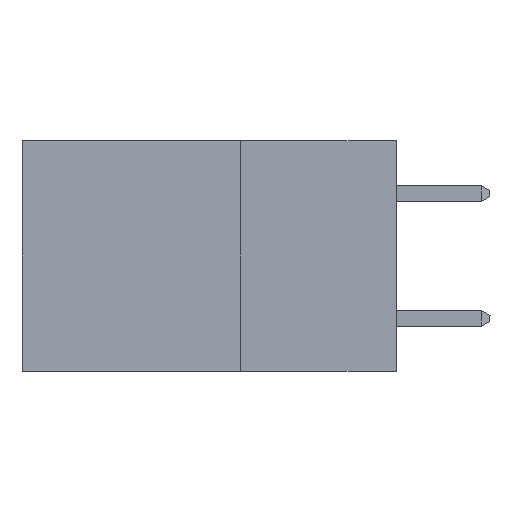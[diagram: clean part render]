
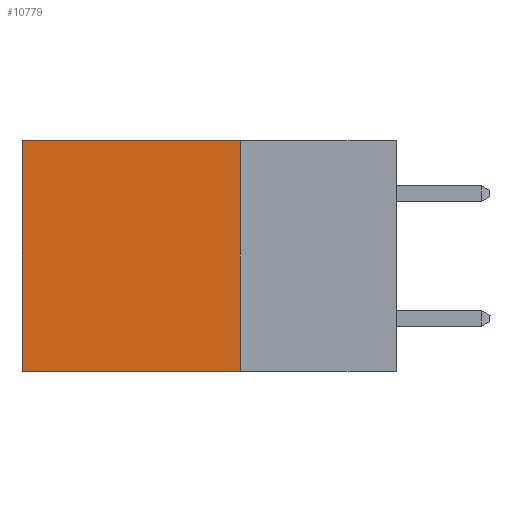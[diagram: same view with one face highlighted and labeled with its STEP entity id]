
A CAD part, left-side view. The second image highlights one B-rep face of the part: STEP entity #10779.
In plain terms, the highlighted planar face has unit normal (-1, 0, 0).
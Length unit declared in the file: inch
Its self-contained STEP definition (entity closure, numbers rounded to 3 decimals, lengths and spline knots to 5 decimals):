
#13 = PLANE ( 'NONE',  #3113 ) ;
#426 = CARTESIAN_POINT ( 'NONE',  ( 0.298, 0.6, 0. ) ) ;
#3113 = AXIS2_PLACEMENT_3D ( 'NONE', #16318, #10113, #12138 ) ;
#3839 = VECTOR ( 'NONE', #6429, 39.37008 ) ;
#4372 = LINE ( 'NONE', #426, #19845 ) ;
#5402 = ORIENTED_EDGE ( 'NONE', *, *, #8547, .F. ) ;
#5595 = VERTEX_POINT ( 'NONE', #21946 ) ;
#5607 = EDGE_CURVE ( 'NONE', #5595, #17374, #20962, .T. ) ;
#6304 = EDGE_LOOP ( 'NONE', ( #10473, #5402, #8585, #14293 ) ) ;
#6429 = DIRECTION ( 'NONE',  ( 0., 1., 0. ) ) ;
#6780 = CARTESIAN_POINT ( 'NONE',  ( 0.298, 0.25, -0.37 ) ) ;
#7233 = FACE_OUTER_BOUND ( 'NONE', #6304, .T. ) ;
#7769 = CARTESIAN_POINT ( 'NONE',  ( 0.298, 0.6, 0. ) ) ;
#8212 = VECTOR ( 'NONE', #14818, 39.37008 ) ;
#8547 = EDGE_CURVE ( 'NONE', #22191, #12712, #25007, .T. ) ;
#8585 = ORIENTED_EDGE ( 'NONE', *, *, #25036, .F. ) ;
#10113 = DIRECTION ( 'NONE',  ( 1., 0., 0. ) ) ;
#10473 = ORIENTED_EDGE ( 'NONE', *, *, #18864, .T. ) ;
#10779 = ADVANCED_FACE ( 'NONE', ( #7233 ), #13, .F. ) ;
#12138 = DIRECTION ( 'NONE',  ( 0., 0., -1. ) ) ;
#12712 = VERTEX_POINT ( 'NONE', #21844 ) ;
#12806 = DIRECTION ( 'NONE',  ( 0., 0., -1. ) ) ;
#12925 = CARTESIAN_POINT ( 'NONE',  ( 0.298, 0.25, 0. ) ) ;
#14293 = ORIENTED_EDGE ( 'NONE', *, *, #5607, .T. ) ;
#14818 = DIRECTION ( 'NONE',  ( 0., 0., -1. ) ) ;
#16318 = CARTESIAN_POINT ( 'NONE',  ( 0.298, 0.25, 0. ) ) ;
#17374 = VERTEX_POINT ( 'NONE', #7769 ) ;
#18864 = EDGE_CURVE ( 'NONE', #17374, #12712, #4372, .T. ) ;
#19832 = DIRECTION ( 'NONE',  ( 0., 1., 0. ) ) ;
#19845 = VECTOR ( 'NONE', #12806, 39.37008 ) ;
#20051 = VECTOR ( 'NONE', #19832, 39.37008 ) ;
#20962 = LINE ( 'NONE', #22131, #20051 ) ;
#21844 = CARTESIAN_POINT ( 'NONE',  ( 0.298, 0.6, -0.37 ) ) ;
#21946 = CARTESIAN_POINT ( 'NONE',  ( 0.298, 0.25, 0. ) ) ;
#22131 = CARTESIAN_POINT ( 'NONE',  ( 0.298, 0.25, 0. ) ) ;
#22191 = VERTEX_POINT ( 'NONE', #26102 ) ;
#25007 = LINE ( 'NONE', #6780, #3839 ) ;
#25036 = EDGE_CURVE ( 'NONE', #5595, #22191, #25872, .T. ) ;
#25872 = LINE ( 'NONE', #12925, #8212 ) ;
#26102 = CARTESIAN_POINT ( 'NONE',  ( 0.298, 0.25, -0.37 ) ) ;
